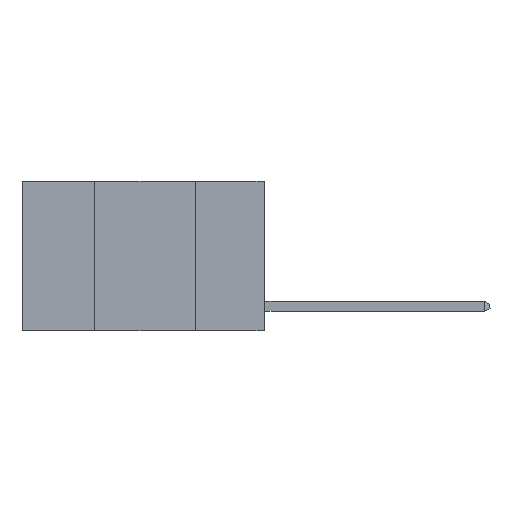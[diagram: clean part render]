
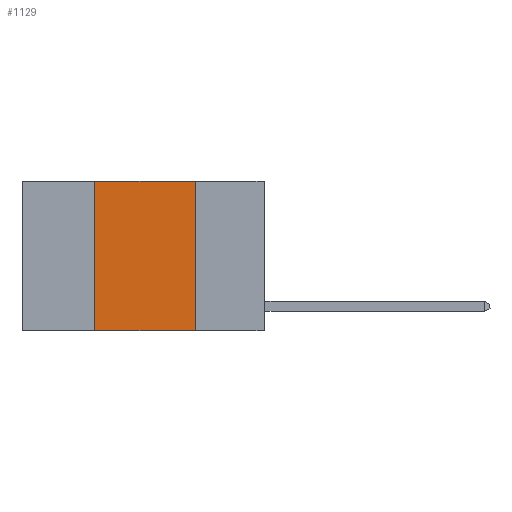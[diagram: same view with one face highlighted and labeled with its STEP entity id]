
A CAD part, left-side view. The second image highlights one B-rep face of the part: STEP entity #1129.
In plain terms, the highlighted planar face has unit normal (-1, 0, 0).
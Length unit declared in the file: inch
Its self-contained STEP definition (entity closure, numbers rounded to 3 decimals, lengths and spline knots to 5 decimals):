
#470 = EDGE_CURVE ( 'NONE', #6171, #1544, #6077, .T. ) ;
#672 = VERTEX_POINT ( 'NONE', #7471 ) ;
#728 = DIRECTION ( 'NONE',  ( 0., 0., -1. ) ) ;
#1129 = ADVANCED_FACE ( 'NONE', ( #3799 ), #9238, .F. ) ;
#1273 = CARTESIAN_POINT ( 'NONE',  ( 0., 0.42, 0. ) ) ;
#1544 = VERTEX_POINT ( 'NONE', #4142 ) ;
#1567 = DIRECTION ( 'NONE',  ( 1., 0., 0. ) ) ;
#1852 = LINE ( 'NONE', #4915, #3099 ) ;
#1868 = DIRECTION ( 'NONE',  ( 0., 0., 1. ) ) ;
#1953 = LINE ( 'NONE', #9597, #7576 ) ;
#2077 = ORIENTED_EDGE ( 'NONE', *, *, #4881, .F. ) ;
#2234 = AXIS2_PLACEMENT_3D ( 'NONE', #8455, #1567, #728 ) ;
#2346 = EDGE_CURVE ( 'NONE', #6765, #6171, #5832, .T. ) ;
#2692 = DIRECTION ( 'NONE',  ( 0., 0., -1. ) ) ;
#2753 = CARTESIAN_POINT ( 'NONE',  ( 0., 0.42, -0.37 ) ) ;
#2822 = ORIENTED_EDGE ( 'NONE', *, *, #470, .F. ) ;
#3099 = VECTOR ( 'NONE', #4587, 39.37008 ) ;
#3367 = EDGE_LOOP ( 'NONE', ( #2077, #2822, #4707, #6350 ) ) ;
#3799 = FACE_OUTER_BOUND ( 'NONE', #3367, .T. ) ;
#4142 = CARTESIAN_POINT ( 'NONE',  ( 0., 0.17, 0. ) ) ;
#4296 = VECTOR ( 'NONE', #1868, 39.37008 ) ;
#4587 = DIRECTION ( 'NONE',  ( 0., -1., 0. ) ) ;
#4664 = CARTESIAN_POINT ( 'NONE',  ( 0., 0.6, 0. ) ) ;
#4707 = ORIENTED_EDGE ( 'NONE', *, *, #2346, .F. ) ;
#4881 = EDGE_CURVE ( 'NONE', #1544, #672, #1953, .T. ) ;
#4915 = CARTESIAN_POINT ( 'NONE',  ( 0., 0.6, -0.37 ) ) ;
#5704 = EDGE_CURVE ( 'NONE', #6765, #672, #1852, .T. ) ;
#5832 = LINE ( 'NONE', #1273, #4296 ) ;
#6077 = LINE ( 'NONE', #4664, #8991 ) ;
#6171 = VERTEX_POINT ( 'NONE', #6826 ) ;
#6350 = ORIENTED_EDGE ( 'NONE', *, *, #5704, .T. ) ;
#6765 = VERTEX_POINT ( 'NONE', #2753 ) ;
#6826 = CARTESIAN_POINT ( 'NONE',  ( 0., 0.42, 0. ) ) ;
#7471 = CARTESIAN_POINT ( 'NONE',  ( 0., 0.17, -0.37 ) ) ;
#7576 = VECTOR ( 'NONE', #2692, 39.37008 ) ;
#8455 = CARTESIAN_POINT ( 'NONE',  ( 0., 0.6, 0. ) ) ;
#8991 = VECTOR ( 'NONE', #9084, 39.37008 ) ;
#9084 = DIRECTION ( 'NONE',  ( 0., -1., 0. ) ) ;
#9238 = PLANE ( 'NONE',  #2234 ) ;
#9597 = CARTESIAN_POINT ( 'NONE',  ( 0., 0.17, 0. ) ) ;
